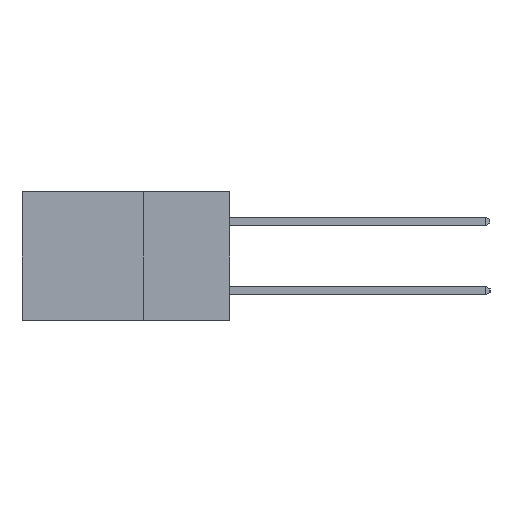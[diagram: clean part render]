
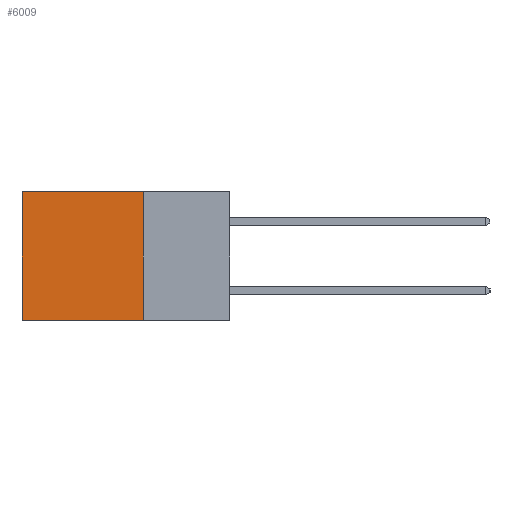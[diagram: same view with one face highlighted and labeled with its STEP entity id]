
A CAD part, left-side view. The second image highlights one B-rep face of the part: STEP entity #6009.
In plain terms, the highlighted planar face has unit normal (-1, 0, 0).
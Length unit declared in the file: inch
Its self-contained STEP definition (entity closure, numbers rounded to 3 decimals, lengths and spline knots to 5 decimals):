
#505 = VERTEX_POINT ( 'NONE', #8590 ) ;
#574 = LINE ( 'NONE', #2887, #3518 ) ;
#1043 = VERTEX_POINT ( 'NONE', #4498 ) ;
#1099 = DIRECTION ( 'NONE',  ( 0., 0., -1. ) ) ;
#1997 = EDGE_CURVE ( 'NONE', #1043, #5221, #5945, .T. ) ;
#2887 = CARTESIAN_POINT ( 'NONE',  ( 0.2615, 0.6, -0.37 ) ) ;
#3104 = CARTESIAN_POINT ( 'NONE',  ( 0.2615, 0.25, 0. ) ) ;
#3234 = PLANE ( 'NONE',  #9596 ) ;
#3285 = CARTESIAN_POINT ( 'NONE',  ( 0.2615, 0.25, -0.37 ) ) ;
#3447 = EDGE_CURVE ( 'NONE', #4726, #505, #11432, .T. ) ;
#3518 = VECTOR ( 'NONE', #3866, 39.37008 ) ;
#3864 = EDGE_CURVE ( 'NONE', #5221, #505, #574, .T. ) ;
#3866 = DIRECTION ( 'NONE',  ( 0., 0., -1. ) ) ;
#4014 = CARTESIAN_POINT ( 'NONE',  ( 0.2615, 0.25, -0.37 ) ) ;
#4189 = DIRECTION ( 'NONE',  ( 0., 0., -1. ) ) ;
#4243 = ORIENTED_EDGE ( 'NONE', *, *, #1997, .T. ) ;
#4498 = CARTESIAN_POINT ( 'NONE',  ( 0.2615, 0.25, 0. ) ) ;
#4653 = EDGE_CURVE ( 'NONE', #1043, #4726, #11548, .T. ) ;
#4726 = VERTEX_POINT ( 'NONE', #6913 ) ;
#5221 = VERTEX_POINT ( 'NONE', #8619 ) ;
#5945 = LINE ( 'NONE', #3104, #10043 ) ;
#6009 = ADVANCED_FACE ( 'NONE', ( #10386 ), #3234, .F. ) ;
#6084 = CARTESIAN_POINT ( 'NONE',  ( 0.2615, 0.25, -0.37 ) ) ;
#6135 = DIRECTION ( 'NONE',  ( 0., 1., 0. ) ) ;
#6164 = ORIENTED_EDGE ( 'NONE', *, *, #3447, .F. ) ;
#6403 = ORIENTED_EDGE ( 'NONE', *, *, #4653, .F. ) ;
#6871 = EDGE_LOOP ( 'NONE', ( #8365, #6164, #6403, #4243 ) ) ;
#6913 = CARTESIAN_POINT ( 'NONE',  ( 0.2615, 0.25, -0.37 ) ) ;
#8365 = ORIENTED_EDGE ( 'NONE', *, *, #3864, .T. ) ;
#8590 = CARTESIAN_POINT ( 'NONE',  ( 0.2615, 0.6, -0.37 ) ) ;
#8619 = CARTESIAN_POINT ( 'NONE',  ( 0.2615, 0.6, 0. ) ) ;
#9104 = VECTOR ( 'NONE', #1099, 39.37008 ) ;
#9275 = VECTOR ( 'NONE', #6135, 39.37008 ) ;
#9596 = AXIS2_PLACEMENT_3D ( 'NONE', #6084, #9834, #4189 ) ;
#9700 = DIRECTION ( 'NONE',  ( 0., 1., 0. ) ) ;
#9834 = DIRECTION ( 'NONE',  ( 1., 0., 0. ) ) ;
#10043 = VECTOR ( 'NONE', #9700, 39.37008 ) ;
#10386 = FACE_OUTER_BOUND ( 'NONE', #6871, .T. ) ;
#11432 = LINE ( 'NONE', #3285, #9275 ) ;
#11548 = LINE ( 'NONE', #4014, #9104 ) ;
